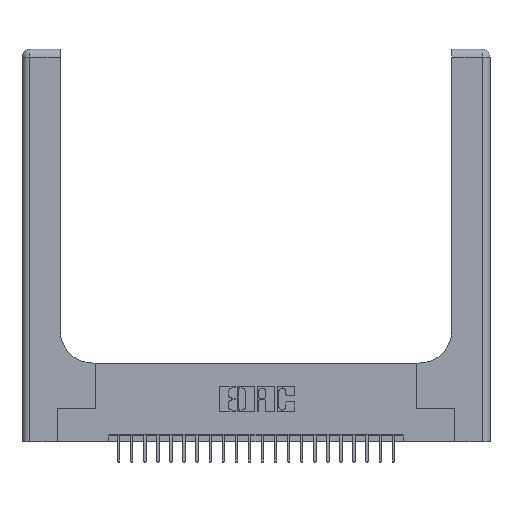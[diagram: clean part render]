
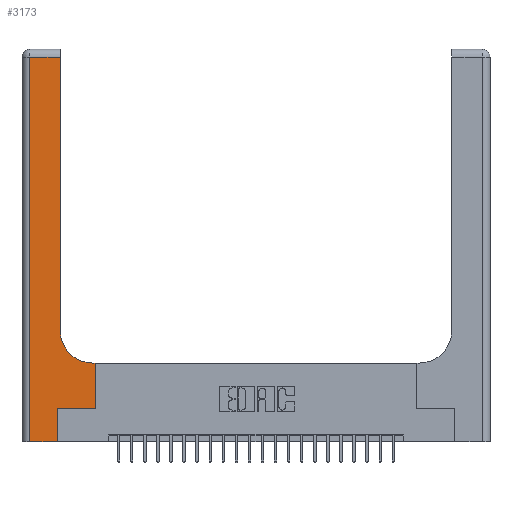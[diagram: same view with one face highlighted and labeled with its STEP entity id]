
A CAD part, top view. The second image highlights one B-rep face of the part: STEP entity #3173.
In plain terms, the highlighted planar face has unit normal (0, 0, 1).
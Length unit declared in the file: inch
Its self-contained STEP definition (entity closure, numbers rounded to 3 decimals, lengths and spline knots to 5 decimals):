
#171 = VERTEX_POINT ( 'NONE', #2942 ) ;
#503 = VECTOR ( 'NONE', #12584, 39.37008 ) ;
#807 = ORIENTED_EDGE ( 'NONE', *, *, #24611, .T. ) ;
#1724 = CARTESIAN_POINT ( 'NONE',  ( 0.5415, 0.6, 0.37 ) ) ;
#1780 = CARTESIAN_POINT ( 'NONE',  ( 0.269, 0.25, 0.37 ) ) ;
#2151 = CARTESIAN_POINT ( 'NONE',  ( 0.269, 0., 0.37 ) ) ;
#2942 = CARTESIAN_POINT ( 'NONE',  ( 0.06, 2.94, 0.37 ) ) ;
#3057 = CARTESIAN_POINT ( 'NONE',  ( 0.5585, 0.6, 0.37 ) ) ;
#3128 = DIRECTION ( 'NONE',  ( 0., 0., -1. ) ) ;
#3173 = ADVANCED_FACE ( 'NONE', ( #14872 ), #6417, .F. ) ;
#3249 = LINE ( 'NONE', #8617, #13122 ) ;
#3534 = VECTOR ( 'NONE', #4226, 39.37008 ) ;
#4226 = DIRECTION ( 'NONE',  ( 0., 1., 0. ) ) ;
#4273 = CARTESIAN_POINT ( 'NONE',  ( 0.5585, 0.25, 0.37 ) ) ;
#5701 = EDGE_CURVE ( 'NONE', #16465, #15879, #8839, .T. ) ;
#5992 = EDGE_CURVE ( 'NONE', #13360, #16400, #17623, .T. ) ;
#6417 = PLANE ( 'NONE',  #24891 ) ;
#6534 = ORIENTED_EDGE ( 'NONE', *, *, #20243, .T. ) ;
#6709 = DIRECTION ( 'NONE',  ( 0., 1., 0. ) ) ;
#7172 = LINE ( 'NONE', #10646, #503 ) ;
#7470 = ORIENTED_EDGE ( 'NONE', *, *, #8499, .T. ) ;
#7563 = VERTEX_POINT ( 'NONE', #15199 ) ;
#7955 = VECTOR ( 'NONE', #6709, 39.37008 ) ;
#8499 = EDGE_CURVE ( 'NONE', #20701, #12178, #15700, .T. ) ;
#8617 = CARTESIAN_POINT ( 'NONE',  ( 0., 2.94, 0.37 ) ) ;
#8839 = LINE ( 'NONE', #2151, #3534 ) ;
#9315 = ORIENTED_EDGE ( 'NONE', *, *, #17016, .T. ) ;
#9335 = VECTOR ( 'NONE', #9779, 39.37008 ) ;
#9779 = DIRECTION ( 'NONE',  ( -1., 0., 0. ) ) ;
#9806 = DIRECTION ( 'NONE',  ( 0., -1., 0. ) ) ;
#10376 = DIRECTION ( 'NONE',  ( 0., 0., -1. ) ) ;
#10646 = CARTESIAN_POINT ( 'NONE',  ( 0.269, 0.25, 0.37 ) ) ;
#10900 = AXIS2_PLACEMENT_3D ( 'NONE', #14923, #3128, #16859 ) ;
#11467 = EDGE_LOOP ( 'NONE', ( #19546, #6534, #22480, #18654, #24836, #807, #7470, #9315, #21341 ) ) ;
#12178 = VERTEX_POINT ( 'NONE', #3057 ) ;
#12526 = DIRECTION ( 'NONE',  ( -1., 0., 0. ) ) ;
#12584 = DIRECTION ( 'NONE',  ( 1., 0., 0. ) ) ;
#13067 = VERTEX_POINT ( 'NONE', #20546 ) ;
#13076 = EDGE_CURVE ( 'NONE', #13067, #16465, #14415, .T. ) ;
#13122 = VECTOR ( 'NONE', #12526, 39.37008 ) ;
#13360 = VERTEX_POINT ( 'NONE', #1724 ) ;
#13940 = CARTESIAN_POINT ( 'NONE',  ( 0.5585, 0.25, 0.37 ) ) ;
#14415 = LINE ( 'NONE', #22414, #24492 ) ;
#14872 = FACE_OUTER_BOUND ( 'NONE', #11467, .T. ) ;
#14923 = CARTESIAN_POINT ( 'NONE',  ( 0.5415, 0.85, 0.37 ) ) ;
#15199 = CARTESIAN_POINT ( 'NONE',  ( 0.2915, 2.94, 0.37 ) ) ;
#15700 = LINE ( 'NONE', #4273, #24551 ) ;
#15879 = VERTEX_POINT ( 'NONE', #1780 ) ;
#16119 = CARTESIAN_POINT ( 'NONE',  ( 0., 3., 0.37 ) ) ;
#16400 = VERTEX_POINT ( 'NONE', #17509 ) ;
#16433 = EDGE_CURVE ( 'NONE', #171, #13067, #23755, .T. ) ;
#16465 = VERTEX_POINT ( 'NONE', #23324 ) ;
#16859 = DIRECTION ( 'NONE',  ( 1., 0., 0. ) ) ;
#17016 = EDGE_CURVE ( 'NONE', #12178, #13360, #24574, .T. ) ;
#17509 = CARTESIAN_POINT ( 'NONE',  ( 0.2915, 0.85, 0.37 ) ) ;
#17623 = CIRCLE ( 'NONE', #10900, 0.25 ) ;
#18234 = LINE ( 'NONE', #20226, #7955 ) ;
#18654 = ORIENTED_EDGE ( 'NONE', *, *, #13076, .T. ) ;
#19476 = CARTESIAN_POINT ( 'NONE',  ( 0.06, 3., 0.37 ) ) ;
#19546 = ORIENTED_EDGE ( 'NONE', *, *, #20262, .T. ) ;
#19821 = DIRECTION ( 'NONE',  ( 0., 1., 0. ) ) ;
#20226 = CARTESIAN_POINT ( 'NONE',  ( 0.2915, 3., 0.37 ) ) ;
#20243 = EDGE_CURVE ( 'NONE', #7563, #171, #3249, .T. ) ;
#20262 = EDGE_CURVE ( 'NONE', #16400, #7563, #18234, .T. ) ;
#20546 = CARTESIAN_POINT ( 'NONE',  ( 0.06, 0., 0.37 ) ) ;
#20701 = VERTEX_POINT ( 'NONE', #13940 ) ;
#21341 = ORIENTED_EDGE ( 'NONE', *, *, #5992, .T. ) ;
#22414 = CARTESIAN_POINT ( 'NONE',  ( 0., 0., 0.37 ) ) ;
#22480 = ORIENTED_EDGE ( 'NONE', *, *, #16433, .T. ) ;
#23136 = CARTESIAN_POINT ( 'NONE',  ( 0.2915, 0.6, 0.37 ) ) ;
#23324 = CARTESIAN_POINT ( 'NONE',  ( 0.269, 0., 0.37 ) ) ;
#23701 = DIRECTION ( 'NONE',  ( -1., 0., 0. ) ) ;
#23755 = LINE ( 'NONE', #19476, #24351 ) ;
#24307 = DIRECTION ( 'NONE',  ( 1., 0., 0. ) ) ;
#24351 = VECTOR ( 'NONE', #9806, 39.37008 ) ;
#24492 = VECTOR ( 'NONE', #24307, 39.37008 ) ;
#24551 = VECTOR ( 'NONE', #19821, 39.37008 ) ;
#24574 = LINE ( 'NONE', #23136, #9335 ) ;
#24611 = EDGE_CURVE ( 'NONE', #15879, #20701, #7172, .T. ) ;
#24836 = ORIENTED_EDGE ( 'NONE', *, *, #5701, .T. ) ;
#24891 = AXIS2_PLACEMENT_3D ( 'NONE', #16119, #10376, #23701 ) ;
